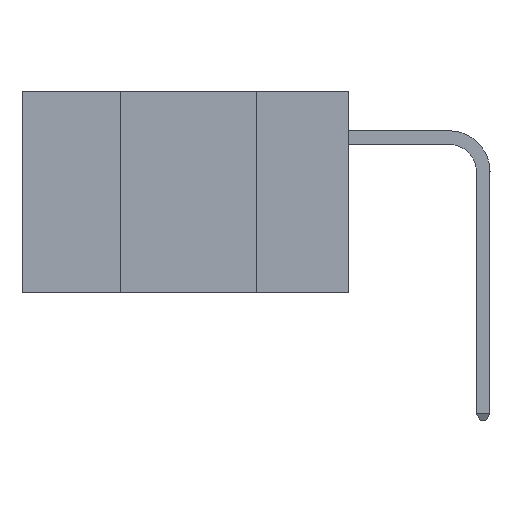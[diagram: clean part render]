
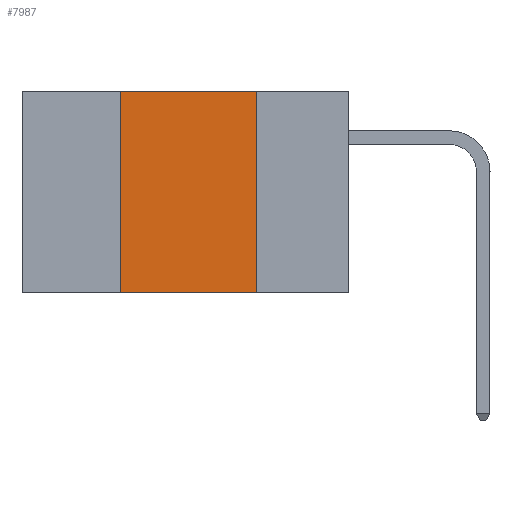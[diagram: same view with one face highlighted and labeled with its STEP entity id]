
A CAD part, left-side view. The second image highlights one B-rep face of the part: STEP entity #7987.
In plain terms, the highlighted planar face has unit normal (-1, 0, 0).
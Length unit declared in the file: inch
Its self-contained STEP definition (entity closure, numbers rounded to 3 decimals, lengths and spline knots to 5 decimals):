
#100 = DIRECTION ( 'NONE',  ( 0., -1., 0. ) ) ;
#186 = CARTESIAN_POINT ( 'NONE',  ( 0., 0.42, -0.37 ) ) ;
#1969 = CARTESIAN_POINT ( 'NONE',  ( 0., 0.42, 0. ) ) ;
#3074 = LINE ( 'NONE', #14706, #3698 ) ;
#3311 = CARTESIAN_POINT ( 'NONE',  ( 0., 0.42, 0. ) ) ;
#3552 = CARTESIAN_POINT ( 'NONE',  ( 0., 0.17, 0. ) ) ;
#3698 = VECTOR ( 'NONE', #16627, 39.37008 ) ;
#3725 = DIRECTION ( 'NONE',  ( 0., -1., 0. ) ) ;
#3910 = ORIENTED_EDGE ( 'NONE', *, *, #20391, .F. ) ;
#3921 = CARTESIAN_POINT ( 'NONE',  ( 0., 0.6, 0. ) ) ;
#4037 = VERTEX_POINT ( 'NONE', #186 ) ;
#4598 = EDGE_CURVE ( 'NONE', #4037, #23510, #12246, .T. ) ;
#5323 = DIRECTION ( 'NONE',  ( 0., 0., 1. ) ) ;
#5330 = CARTESIAN_POINT ( 'NONE',  ( 0., 0.6, 0. ) ) ;
#6387 = VERTEX_POINT ( 'NONE', #3552 ) ;
#7336 = DIRECTION ( 'NONE',  ( 1., 0., 0. ) ) ;
#7682 = VECTOR ( 'NONE', #5323, 39.37008 ) ;
#7987 = ADVANCED_FACE ( 'NONE', ( #10074 ), #16915, .F. ) ;
#9119 = VECTOR ( 'NONE', #100, 39.37008 ) ;
#9723 = CARTESIAN_POINT ( 'NONE',  ( 0., 0.6, -0.37 ) ) ;
#10074 = FACE_OUTER_BOUND ( 'NONE', #21666, .T. ) ;
#12246 = LINE ( 'NONE', #9723, #22369 ) ;
#14193 = LINE ( 'NONE', #3921, #9119 ) ;
#14281 = ORIENTED_EDGE ( 'NONE', *, *, #24385, .F. ) ;
#14706 = CARTESIAN_POINT ( 'NONE',  ( 0., 0.17, 0. ) ) ;
#14878 = ORIENTED_EDGE ( 'NONE', *, *, #4598, .T. ) ;
#16627 = DIRECTION ( 'NONE',  ( 0., 0., -1. ) ) ;
#16915 = PLANE ( 'NONE',  #21400 ) ;
#18459 = LINE ( 'NONE', #3311, #7682 ) ;
#20391 = EDGE_CURVE ( 'NONE', #22762, #6387, #14193, .T. ) ;
#20709 = DIRECTION ( 'NONE',  ( 0., 0., -1. ) ) ;
#21400 = AXIS2_PLACEMENT_3D ( 'NONE', #5330, #7336, #20709 ) ;
#21666 = EDGE_LOOP ( 'NONE', ( #23173, #3910, #14281, #14878 ) ) ;
#22369 = VECTOR ( 'NONE', #3725, 39.37008 ) ;
#22762 = VERTEX_POINT ( 'NONE', #1969 ) ;
#23098 = EDGE_CURVE ( 'NONE', #6387, #23510, #3074, .T. ) ;
#23173 = ORIENTED_EDGE ( 'NONE', *, *, #23098, .F. ) ;
#23510 = VERTEX_POINT ( 'NONE', #23888 ) ;
#23888 = CARTESIAN_POINT ( 'NONE',  ( 0., 0.17, -0.37 ) ) ;
#24385 = EDGE_CURVE ( 'NONE', #4037, #22762, #18459, .T. ) ;
